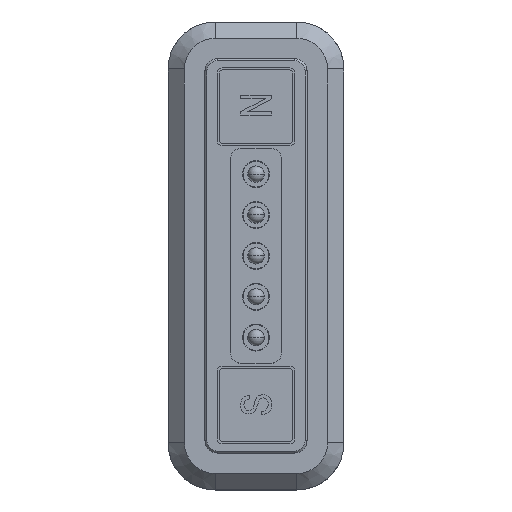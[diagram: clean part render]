
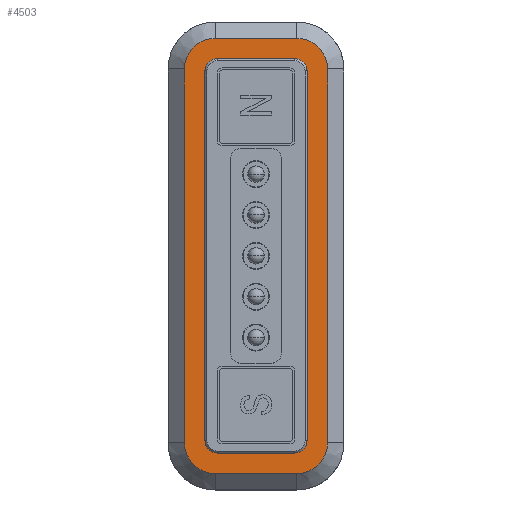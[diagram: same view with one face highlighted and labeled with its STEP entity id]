
A CAD part, top view. The second image highlights one B-rep face of the part: STEP entity #4503.
In plain terms, the highlighted planar face has unit normal (0, 0, 1).
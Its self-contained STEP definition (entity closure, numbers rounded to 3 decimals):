
#273 = LINE ( 'NONE', #8323, #10789 ) ;
#417 = DIRECTION ( 'NONE',  ( 0., 1., 0. ) ) ;
#451 = DIRECTION ( 'NONE',  ( 0., 0., 1. ) ) ;
#462 = AXIS2_PLACEMENT_3D ( 'NONE', #3428, #12684, #9722 ) ;
#503 = LINE ( 'NONE', #6586, #4382 ) ;
#523 = CARTESIAN_POINT ( 'NONE',  ( -2., -9.15, 2. ) ) ;
#628 = EDGE_CURVE ( 'NONE', #7473, #11965, #1548, .T. ) ;
#861 = VERTEX_POINT ( 'NONE', #5571 ) ;
#894 = CIRCLE ( 'NONE', #5940, 0.6 ) ;
#910 = EDGE_CURVE ( 'NONE', #11567, #2039, #5899, .T. ) ;
#1056 = LINE ( 'NONE', #11018, #11664 ) ;
#1071 = DIRECTION ( 'NONE',  ( 1., 0., 0. ) ) ;
#1141 = VERTEX_POINT ( 'NONE', #12849 ) ;
#1163 = CARTESIAN_POINT ( 'NONE',  ( -2., -10.65, 2. ) ) ;
#1347 = EDGE_CURVE ( 'NONE', #12868, #2146, #6434, .T. ) ;
#1359 = CARTESIAN_POINT ( 'NONE',  ( -2.5, 9.05, 2. ) ) ;
#1430 = VERTEX_POINT ( 'NONE', #4638 ) ;
#1497 = CARTESIAN_POINT ( 'NONE',  ( -2.5, 9.05, 2. ) ) ;
#1548 = CIRCLE ( 'NONE', #5971, 0.6 ) ;
#1587 = FACE_OUTER_BOUND ( 'NONE', #8108, .T. ) ;
#1721 = FACE_BOUND ( 'NONE', #8053, .T. ) ;
#1758 = CARTESIAN_POINT ( 'NONE',  ( -3.5, -9.15, 2. ) ) ;
#1956 = CIRCLE ( 'NONE', #7018, 0.6 ) ;
#2027 = ORIENTED_EDGE ( 'NONE', *, *, #7537, .T. ) ;
#2039 = VERTEX_POINT ( 'NONE', #9531 ) ;
#2071 = ORIENTED_EDGE ( 'NONE', *, *, #6403, .F. ) ;
#2143 = DIRECTION ( 'NONE',  ( 0., 0., 1. ) ) ;
#2146 = VERTEX_POINT ( 'NONE', #6118 ) ;
#2156 = DIRECTION ( 'NONE',  ( -1., 0., 0. ) ) ;
#2230 = ORIENTED_EDGE ( 'NONE', *, *, #6469, .F. ) ;
#2301 = DIRECTION ( 'NONE',  ( -1., 0., 0. ) ) ;
#2375 = VERTEX_POINT ( 'NONE', #11819 ) ;
#2395 = VERTEX_POINT ( 'NONE', #12066 ) ;
#2510 = ORIENTED_EDGE ( 'NONE', *, *, #628, .F. ) ;
#2610 = CARTESIAN_POINT ( 'NONE',  ( 2.5, -9.05, 2. ) ) ;
#2690 = AXIS2_PLACEMENT_3D ( 'NONE', #10380, #2143, #1071 ) ;
#2801 = DIRECTION ( 'NONE',  ( 0., -1., 0. ) ) ;
#3428 = CARTESIAN_POINT ( 'NONE',  ( 2., -9.15, 2. ) ) ;
#3467 = ORIENTED_EDGE ( 'NONE', *, *, #7705, .T. ) ;
#3516 = CARTESIAN_POINT ( 'NONE',  ( -1.9, -9.65, 2. ) ) ;
#3520 = DIRECTION ( 'NONE',  ( -1., 0., 0. ) ) ;
#3756 = AXIS2_PLACEMENT_3D ( 'NONE', #6052, #5132, #2156 ) ;
#3759 = DIRECTION ( 'NONE',  ( -1., 0., 0. ) ) ;
#3814 = CARTESIAN_POINT ( 'NONE',  ( 3.5, -9.15, 2. ) ) ;
#4150 = ORIENTED_EDGE ( 'NONE', *, *, #8838, .T. ) ;
#4195 = EDGE_CURVE ( 'NONE', #2375, #2395, #7151, .T. ) ;
#4382 = VECTOR ( 'NONE', #5592, 1000. ) ;
#4503 = ADVANCED_FACE ( 'NONE', ( #1587, #1721 ), #11726, .F. ) ;
#4638 = CARTESIAN_POINT ( 'NONE',  ( 1.9, -9.65, 2. ) ) ;
#4671 = VECTOR ( 'NONE', #8360, 1000. ) ;
#5132 = DIRECTION ( 'NONE',  ( 0., 0., 1. ) ) ;
#5195 = DIRECTION ( 'NONE',  ( 1., 0., 0. ) ) ;
#5316 = ORIENTED_EDGE ( 'NONE', *, *, #10620, .T. ) ;
#5442 = CARTESIAN_POINT ( 'NONE',  ( 2.5, 9.05, 2. ) ) ;
#5571 = CARTESIAN_POINT ( 'NONE',  ( -3.5, -9.15, 2. ) ) ;
#5577 = CARTESIAN_POINT ( 'NONE',  ( -2.5, -9.05, 2. ) ) ;
#5592 = DIRECTION ( 'NONE',  ( -1., 0., 0. ) ) ;
#5827 = CARTESIAN_POINT ( 'NONE',  ( 2., -10.65, 2. ) ) ;
#5899 = LINE ( 'NONE', #5827, #11192 ) ;
#5940 = AXIS2_PLACEMENT_3D ( 'NONE', #8554, #6574, #12804 ) ;
#5971 = AXIS2_PLACEMENT_3D ( 'NONE', #8330, #11441, #12401 ) ;
#6027 = ORIENTED_EDGE ( 'NONE', *, *, #4195, .T. ) ;
#6052 = CARTESIAN_POINT ( 'NONE',  ( -2., 9.15, 2. ) ) ;
#6118 = CARTESIAN_POINT ( 'NONE',  ( 2.5, 9.05, 2. ) ) ;
#6311 = VERTEX_POINT ( 'NONE', #3814 ) ;
#6403 = EDGE_CURVE ( 'NONE', #11965, #8445, #10467, .T. ) ;
#6434 = LINE ( 'NONE', #5442, #7708 ) ;
#6469 = EDGE_CURVE ( 'NONE', #1430, #12868, #894, .T. ) ;
#6574 = DIRECTION ( 'NONE',  ( 0., 0., 1. ) ) ;
#6586 = CARTESIAN_POINT ( 'NONE',  ( -1.9, 9.65, 2. ) ) ;
#6704 = EDGE_CURVE ( 'NONE', #1141, #2375, #8468, .T. ) ;
#6803 = CIRCLE ( 'NONE', #462, 1.5 ) ;
#6805 = VECTOR ( 'NONE', #3520, 1000. ) ;
#6961 = ORIENTED_EDGE ( 'NONE', *, *, #8109, .F. ) ;
#7018 = AXIS2_PLACEMENT_3D ( 'NONE', #9376, #9310, #5195 ) ;
#7151 = CIRCLE ( 'NONE', #3756, 1.5 ) ;
#7270 = CARTESIAN_POINT ( 'NONE',  ( -1.9, 9.65, 2. ) ) ;
#7306 = AXIS2_PLACEMENT_3D ( 'NONE', #8580, #12834, #3759 ) ;
#7473 = VERTEX_POINT ( 'NONE', #7270 ) ;
#7537 = EDGE_CURVE ( 'NONE', #2039, #6311, #6803, .T. ) ;
#7631 = ORIENTED_EDGE ( 'NONE', *, *, #8532, .F. ) ;
#7636 = ORIENTED_EDGE ( 'NONE', *, *, #10621, .F. ) ;
#7640 = CIRCLE ( 'NONE', #11058, 1.5 ) ;
#7705 = EDGE_CURVE ( 'NONE', #2395, #861, #12073, .T. ) ;
#7708 = VECTOR ( 'NONE', #417, 1000. ) ;
#7891 = VERTEX_POINT ( 'NONE', #3516 ) ;
#8053 = EDGE_LOOP ( 'NONE', ( #7636, #2071, #2510, #6961, #7631, #8475, #2230, #9267 ) ) ;
#8108 = EDGE_LOOP ( 'NONE', ( #6027, #3467, #4150, #11770, #2027, #10816, #5316, #12056 ) ) ;
#8109 = EDGE_CURVE ( 'NONE', #8741, #7473, #503, .T. ) ;
#8323 = CARTESIAN_POINT ( 'NONE',  ( 3.5, -9.15, 2. ) ) ;
#8330 = CARTESIAN_POINT ( 'NONE',  ( -1.9, 9.05, 2. ) ) ;
#8360 = DIRECTION ( 'NONE',  ( 0., -1., 0. ) ) ;
#8445 = VERTEX_POINT ( 'NONE', #5577 ) ;
#8468 = LINE ( 'NONE', #11679, #6805 ) ;
#8475 = ORIENTED_EDGE ( 'NONE', *, *, #1347, .F. ) ;
#8532 = EDGE_CURVE ( 'NONE', #2146, #8741, #13059, .T. ) ;
#8554 = CARTESIAN_POINT ( 'NONE',  ( 1.9, -9.05, 2. ) ) ;
#8580 = CARTESIAN_POINT ( 'NONE',  ( 2., -9.15, 2. ) ) ;
#8609 = CIRCLE ( 'NONE', #9052, 1.5 ) ;
#8741 = VERTEX_POINT ( 'NONE', #12195 ) ;
#8745 = DIRECTION ( 'NONE',  ( 1., 0., 0. ) ) ;
#8838 = EDGE_CURVE ( 'NONE', #861, #11567, #8609, .T. ) ;
#9052 = AXIS2_PLACEMENT_3D ( 'NONE', #523, #451, #10431 ) ;
#9267 = ORIENTED_EDGE ( 'NONE', *, *, #10114, .F. ) ;
#9310 = DIRECTION ( 'NONE',  ( 0., 0., 1. ) ) ;
#9376 = CARTESIAN_POINT ( 'NONE',  ( -1.9, -9.05, 2. ) ) ;
#9531 = CARTESIAN_POINT ( 'NONE',  ( 2., -10.65, 2. ) ) ;
#9722 = DIRECTION ( 'NONE',  ( -1., 0., 0. ) ) ;
#10114 = EDGE_CURVE ( 'NONE', #7891, #1430, #1056, .T. ) ;
#10333 = DIRECTION ( 'NONE',  ( 0., 0., 1. ) ) ;
#10380 = CARTESIAN_POINT ( 'NONE',  ( 1.9, 9.05, 2. ) ) ;
#10431 = DIRECTION ( 'NONE',  ( -1., 0., 0. ) ) ;
#10467 = LINE ( 'NONE', #1359, #4671 ) ;
#10620 = EDGE_CURVE ( 'NONE', #12638, #1141, #7640, .T. ) ;
#10621 = EDGE_CURVE ( 'NONE', #8445, #7891, #1956, .T. ) ;
#10789 = VECTOR ( 'NONE', #12395, 1000. ) ;
#10816 = ORIENTED_EDGE ( 'NONE', *, *, #12472, .T. ) ;
#11018 = CARTESIAN_POINT ( 'NONE',  ( -1.9, -9.65, 2. ) ) ;
#11058 = AXIS2_PLACEMENT_3D ( 'NONE', #11399, #10333, #2301 ) ;
#11192 = VECTOR ( 'NONE', #8745, 1000. ) ;
#11399 = CARTESIAN_POINT ( 'NONE',  ( 2., 9.15, 2. ) ) ;
#11441 = DIRECTION ( 'NONE',  ( 0., 0., 1. ) ) ;
#11567 = VERTEX_POINT ( 'NONE', #1163 ) ;
#11664 = VECTOR ( 'NONE', #12990, 1000. ) ;
#11679 = CARTESIAN_POINT ( 'NONE',  ( -2., 10.65, 2. ) ) ;
#11726 = PLANE ( 'NONE',  #7306 ) ;
#11770 = ORIENTED_EDGE ( 'NONE', *, *, #910, .T. ) ;
#11819 = CARTESIAN_POINT ( 'NONE',  ( -2., 10.65, 2. ) ) ;
#11965 = VERTEX_POINT ( 'NONE', #1497 ) ;
#12056 = ORIENTED_EDGE ( 'NONE', *, *, #6704, .T. ) ;
#12066 = CARTESIAN_POINT ( 'NONE',  ( -3.5, 9.15, 2. ) ) ;
#12073 = LINE ( 'NONE', #1758, #12400 ) ;
#12195 = CARTESIAN_POINT ( 'NONE',  ( 1.9, 9.65, 2. ) ) ;
#12395 = DIRECTION ( 'NONE',  ( 0., 1., 0. ) ) ;
#12400 = VECTOR ( 'NONE', #2801, 1000. ) ;
#12401 = DIRECTION ( 'NONE',  ( 1., 0., 0. ) ) ;
#12472 = EDGE_CURVE ( 'NONE', #6311, #12638, #273, .T. ) ;
#12638 = VERTEX_POINT ( 'NONE', #12768 ) ;
#12684 = DIRECTION ( 'NONE',  ( 0., 0., 1. ) ) ;
#12768 = CARTESIAN_POINT ( 'NONE',  ( 3.5, 9.15, 2. ) ) ;
#12804 = DIRECTION ( 'NONE',  ( -1., 0., 0. ) ) ;
#12834 = DIRECTION ( 'NONE',  ( 0., 0., -1. ) ) ;
#12849 = CARTESIAN_POINT ( 'NONE',  ( 2., 10.65, 2. ) ) ;
#12868 = VERTEX_POINT ( 'NONE', #2610 ) ;
#12990 = DIRECTION ( 'NONE',  ( 1., 0., 0. ) ) ;
#13059 = CIRCLE ( 'NONE', #2690, 0.6 ) ;
